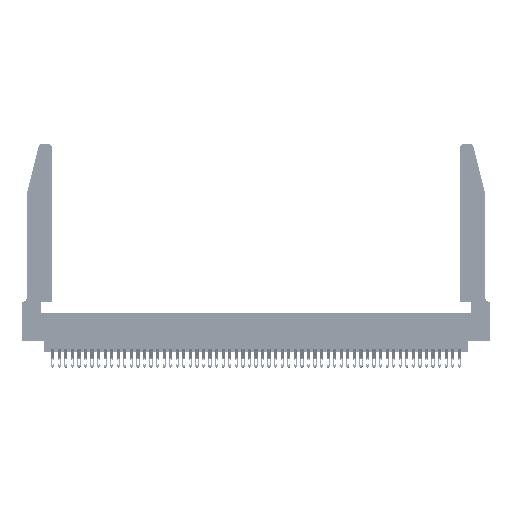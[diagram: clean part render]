
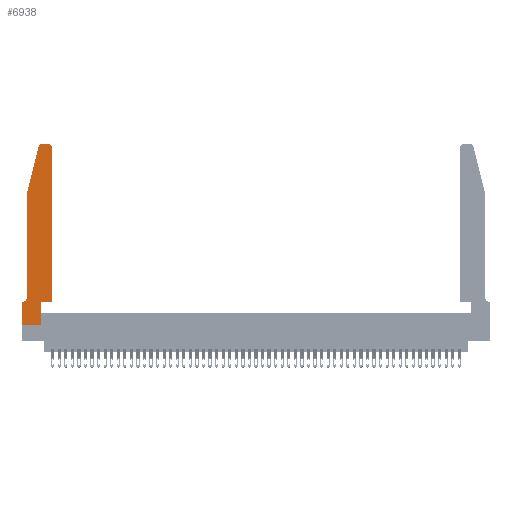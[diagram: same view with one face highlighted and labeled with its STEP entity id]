
A CAD part, top view. The second image highlights one B-rep face of the part: STEP entity #6938.
In plain terms, the highlighted planar face has unit normal (0, 0, 1).
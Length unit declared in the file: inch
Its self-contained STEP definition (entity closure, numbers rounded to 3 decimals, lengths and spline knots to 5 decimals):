
#230 = VECTOR ( 'NONE', #24061, 39.37008 ) ;
#387 = VECTOR ( 'NONE', #39396, 39.37008 ) ;
#627 = DIRECTION ( 'NONE',  ( 1., 0., 0. ) ) ;
#2196 = CIRCLE ( 'NONE', #35567, 0.07 ) ;
#2251 = EDGE_CURVE ( 'NONE', #10199, #48560, #21878, .T. ) ;
#2955 = ORIENTED_EDGE ( 'NONE', *, *, #10280, .T. ) ;
#3534 = CARTESIAN_POINT ( 'NONE',  ( 0.284, 2.75, 0.37 ) ) ;
#3541 = DIRECTION ( 'NONE',  ( 1., 0., 0. ) ) ;
#3739 = EDGE_CURVE ( 'NONE', #39236, #37001, #3858, .T. ) ;
#3744 = EDGE_CURVE ( 'NONE', #37001, #7010, #39564, .T. ) ;
#3858 = LINE ( 'NONE', #8344, #35824 ) ;
#5430 = EDGE_CURVE ( 'NONE', #24601, #39236, #29400, .T. ) ;
#5524 = DIRECTION ( 'NONE',  ( 1., 0., 0. ) ) ;
#6938 = ADVANCED_FACE ( 'NONE', ( #29854 ), #38194, .T. ) ;
#7010 = VERTEX_POINT ( 'NONE', #26910 ) ;
#7732 = EDGE_CURVE ( 'NONE', #35347, #44430, #2196, .T. ) ;
#8344 = CARTESIAN_POINT ( 'NONE',  ( 0.2865, 0.35, 0.37 ) ) ;
#9267 = EDGE_CURVE ( 'NONE', #7010, #38966, #38034, .T. ) ;
#9474 = VERTEX_POINT ( 'NONE', #11858 ) ;
#9772 = CARTESIAN_POINT ( 'NONE',  ( 0.4505, 0.35, 0.37 ) ) ;
#10199 = VERTEX_POINT ( 'NONE', #3534 ) ;
#10280 = EDGE_CURVE ( 'NONE', #9474, #10199, #16081, .T. ) ;
#11462 = CARTESIAN_POINT ( 'NONE',  ( 0.2605, 2.75, 0.37 ) ) ;
#11718 = DIRECTION ( 'NONE',  ( 0., 0., 1. ) ) ;
#11858 = CARTESIAN_POINT ( 'NONE',  ( 0.4205, 2.75, 0.37 ) ) ;
#13070 = DIRECTION ( 'NONE',  ( 0., 0., -1. ) ) ;
#13390 = CARTESIAN_POINT ( 'NONE',  ( 0., 0.35, 0.37 ) ) ;
#13689 = ORIENTED_EDGE ( 'NONE', *, *, #5430, .T. ) ;
#15118 = AXIS2_PLACEMENT_3D ( 'NONE', #35678, #11718, #24677 ) ;
#15342 = CARTESIAN_POINT ( 'NONE',  ( 0.0755, 0.35, 0.37 ) ) ;
#16081 = LINE ( 'NONE', #11462, #387 ) ;
#16763 = CARTESIAN_POINT ( 'NONE',  ( 0.4505, 0.35, 0.37 ) ) ;
#16800 = DIRECTION ( 'NONE',  ( 1., 0., 0. ) ) ;
#17750 = LINE ( 'NONE', #39582, #230 ) ;
#17828 = AXIS2_PLACEMENT_3D ( 'NONE', #34563, #39405, #3541 ) ;
#18316 = CARTESIAN_POINT ( 'NONE',  ( 0.0755, 0.42, 0.37 ) ) ;
#18606 = ORIENTED_EDGE ( 'NONE', *, *, #24335, .T. ) ;
#19335 = AXIS2_PLACEMENT_3D ( 'NONE', #37373, #33721, #5524 ) ;
#19443 = CARTESIAN_POINT ( 'NONE',  ( 0.2865, 0., 0.37 ) ) ;
#19644 = VECTOR ( 'NONE', #26554, 39.37008 ) ;
#19920 = VECTOR ( 'NONE', #47185, 39.37008 ) ;
#21180 = VECTOR ( 'NONE', #37734, 39.37008 ) ;
#21623 = CARTESIAN_POINT ( 'NONE',  ( 0., 0., 0.37 ) ) ;
#21878 = CIRCLE ( 'NONE', #19335, 0.03 ) ;
#22982 = EDGE_CURVE ( 'NONE', #44430, #47435, #39898, .T. ) ;
#24061 = DIRECTION ( 'NONE',  ( 0., -1., 0. ) ) ;
#24335 = EDGE_CURVE ( 'NONE', #51748, #35347, #47916, .T. ) ;
#24540 = ORIENTED_EDGE ( 'NONE', *, *, #22982, .T. ) ;
#24601 = VERTEX_POINT ( 'NONE', #21623 ) ;
#24677 = DIRECTION ( 'NONE',  ( 1., 0., 0. ) ) ;
#25772 = CARTESIAN_POINT ( 'NONE',  ( 0.4505, 2.72, 0.37 ) ) ;
#26554 = DIRECTION ( 'NONE',  ( -0.239, -0.971, 0. ) ) ;
#26910 = CARTESIAN_POINT ( 'NONE',  ( 0.4505, 0.35, 0.37 ) ) ;
#27723 = VECTOR ( 'NONE', #627, 39.37008 ) ;
#27782 = EDGE_LOOP ( 'NONE', ( #2955, #42816, #30016, #18606, #28320, #24540, #47791, #13689, #48707, #29417, #35274, #51075 ) ) ;
#28320 = ORIENTED_EDGE ( 'NONE', *, *, #7732, .T. ) ;
#29058 = LINE ( 'NONE', #34736, #19644 ) ;
#29065 = CARTESIAN_POINT ( 'NONE',  ( 0.25487, 2.72718, 0.37 ) ) ;
#29400 = LINE ( 'NONE', #48466, #43755 ) ;
#29417 = ORIENTED_EDGE ( 'NONE', *, *, #3744, .T. ) ;
#29527 = CARTESIAN_POINT ( 'NONE',  ( 0.0755, 2., 0.37 ) ) ;
#29854 = FACE_OUTER_BOUND ( 'NONE', #27782, .T. ) ;
#30016 = ORIENTED_EDGE ( 'NONE', *, *, #35214, .T. ) ;
#32520 = CARTESIAN_POINT ( 'NONE',  ( 0.0055, 0.42, 0.37 ) ) ;
#32730 = CIRCLE ( 'NONE', #15118, 0.03 ) ;
#33721 = DIRECTION ( 'NONE',  ( 0., 0., 1. ) ) ;
#34563 = CARTESIAN_POINT ( 'NONE',  ( 0., 0.35, 0.37 ) ) ;
#34736 = CARTESIAN_POINT ( 'NONE',  ( 0.0755, 2., 0.37 ) ) ;
#35214 = EDGE_CURVE ( 'NONE', #48560, #51748, #29058, .T. ) ;
#35274 = ORIENTED_EDGE ( 'NONE', *, *, #9267, .T. ) ;
#35347 = VERTEX_POINT ( 'NONE', #18316 ) ;
#35567 = AXIS2_PLACEMENT_3D ( 'NONE', #32520, #13070, #40531 ) ;
#35678 = CARTESIAN_POINT ( 'NONE',  ( 0.4205, 2.72, 0.37 ) ) ;
#35824 = VECTOR ( 'NONE', #36335, 39.37008 ) ;
#36335 = DIRECTION ( 'NONE',  ( 0., 1., 0. ) ) ;
#37001 = VERTEX_POINT ( 'NONE', #42899 ) ;
#37373 = CARTESIAN_POINT ( 'NONE',  ( 0.284, 2.72, 0.37 ) ) ;
#37734 = DIRECTION ( 'NONE',  ( 0., 1., 0. ) ) ;
#38034 = LINE ( 'NONE', #9772, #21180 ) ;
#38194 = PLANE ( 'NONE',  #17828 ) ;
#38966 = VERTEX_POINT ( 'NONE', #25772 ) ;
#39236 = VERTEX_POINT ( 'NONE', #19443 ) ;
#39396 = DIRECTION ( 'NONE',  ( -1., 0., 0. ) ) ;
#39405 = DIRECTION ( 'NONE',  ( 0., 0., 1. ) ) ;
#39438 = DIRECTION ( 'NONE',  ( 0., -1., 0. ) ) ;
#39456 = EDGE_CURVE ( 'NONE', #38966, #9474, #32730, .T. ) ;
#39564 = LINE ( 'NONE', #16763, #27723 ) ;
#39582 = CARTESIAN_POINT ( 'NONE',  ( 0., 0., 0.37 ) ) ;
#39898 = LINE ( 'NONE', #15342, #19920 ) ;
#40395 = CARTESIAN_POINT ( 'NONE',  ( 0.0755, 2., 0.37 ) ) ;
#40531 = DIRECTION ( 'NONE',  ( -1., 0., 0. ) ) ;
#42816 = ORIENTED_EDGE ( 'NONE', *, *, #2251, .T. ) ;
#42899 = CARTESIAN_POINT ( 'NONE',  ( 0.2865, 0.35, 0.37 ) ) ;
#43755 = VECTOR ( 'NONE', #16800, 39.37008 ) ;
#44430 = VERTEX_POINT ( 'NONE', #48426 ) ;
#47185 = DIRECTION ( 'NONE',  ( -1., 0., 0. ) ) ;
#47435 = VERTEX_POINT ( 'NONE', #13390 ) ;
#47791 = ORIENTED_EDGE ( 'NONE', *, *, #50210, .T. ) ;
#47916 = LINE ( 'NONE', #40395, #49177 ) ;
#48426 = CARTESIAN_POINT ( 'NONE',  ( 0.0055, 0.35, 0.37 ) ) ;
#48466 = CARTESIAN_POINT ( 'NONE',  ( 0., 0., 0.37 ) ) ;
#48560 = VERTEX_POINT ( 'NONE', #29065 ) ;
#48707 = ORIENTED_EDGE ( 'NONE', *, *, #3739, .T. ) ;
#49177 = VECTOR ( 'NONE', #39438, 39.37008 ) ;
#50210 = EDGE_CURVE ( 'NONE', #47435, #24601, #17750, .T. ) ;
#51075 = ORIENTED_EDGE ( 'NONE', *, *, #39456, .T. ) ;
#51748 = VERTEX_POINT ( 'NONE', #29527 ) ;
